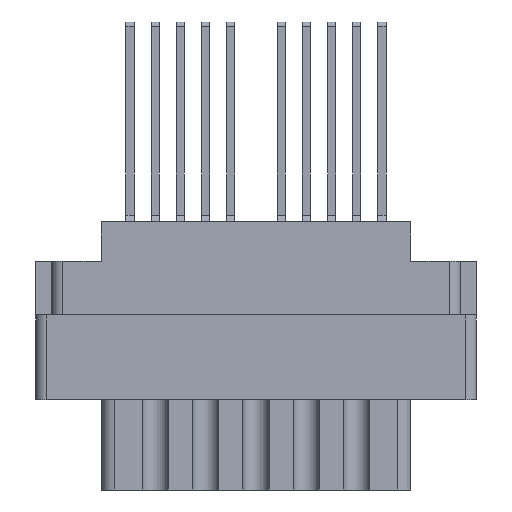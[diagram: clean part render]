
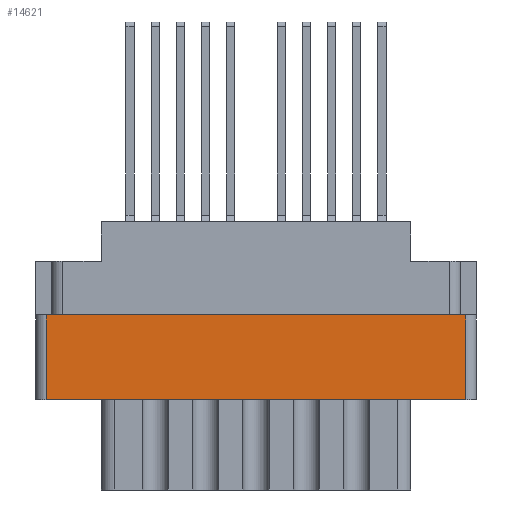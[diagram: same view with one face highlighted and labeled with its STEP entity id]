
A CAD part, front view. The second image highlights one B-rep face of the part: STEP entity #14621.
In plain terms, the highlighted planar face has unit normal (0, -1, 0).
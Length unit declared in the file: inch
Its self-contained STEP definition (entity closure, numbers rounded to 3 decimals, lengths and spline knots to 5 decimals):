
#235 = DIRECTION ( 'NONE',  ( 0., 0., -1. ) ) ;
#299 = CARTESIAN_POINT ( 'NONE',  ( -0.656, -0.343, -0.798 ) ) ;
#824 = LINE ( 'NONE', #15905, #17230 ) ;
#997 = CARTESIAN_POINT ( 'NONE',  ( 0., -0.343, -0.529 ) ) ;
#1767 = EDGE_CURVE ( 'NONE', #13607, #14368, #11355, .T. ) ;
#5175 = EDGE_CURVE ( 'NONE', #15031, #14368, #824, .T. ) ;
#5725 = CARTESIAN_POINT ( 'NONE',  ( -0.624, -0.343, -0.798 ) ) ;
#5846 = VERTEX_POINT ( 'NONE', #23834 ) ;
#6836 = CARTESIAN_POINT ( 'NONE',  ( 0.624, -0.343, -0.798 ) ) ;
#8464 = EDGE_CURVE ( 'NONE', #15031, #5846, #18530, .T. ) ;
#8660 = ORIENTED_EDGE ( 'NONE', *, *, #8464, .T. ) ;
#8854 = ORIENTED_EDGE ( 'NONE', *, *, #1767, .T. ) ;
#9224 = CARTESIAN_POINT ( 'NONE',  ( 0.624, -0.343, -0.529 ) ) ;
#9643 = PLANE ( 'NONE',  #15243 ) ;
#11355 = LINE ( 'NONE', #6836, #15380 ) ;
#12341 = DIRECTION ( 'NONE',  ( 1., 0., 0. ) ) ;
#13358 = VECTOR ( 'NONE', #235, 39.37008 ) ;
#13607 = VERTEX_POINT ( 'NONE', #9224 ) ;
#14368 = VERTEX_POINT ( 'NONE', #23073 ) ;
#14621 = ADVANCED_FACE ( 'NONE', ( #20076 ), #9643, .T. ) ;
#15031 = VERTEX_POINT ( 'NONE', #17907 ) ;
#15243 = AXIS2_PLACEMENT_3D ( 'NONE', #299, #16798, #16959 ) ;
#15380 = VECTOR ( 'NONE', #21464, 39.37008 ) ;
#15501 = EDGE_CURVE ( 'NONE', #13607, #5846, #19212, .T. ) ;
#15905 = CARTESIAN_POINT ( 'NONE',  ( 0., -0.343, -0.277 ) ) ;
#16798 = DIRECTION ( 'NONE',  ( 0., -1., 0. ) ) ;
#16959 = DIRECTION ( 'NONE',  ( 0., 0., -1. ) ) ;
#17141 = ORIENTED_EDGE ( 'NONE', *, *, #5175, .F. ) ;
#17230 = VECTOR ( 'NONE', #12341, 39.37008 ) ;
#17473 = VECTOR ( 'NONE', #19638, 39.37008 ) ;
#17907 = CARTESIAN_POINT ( 'NONE',  ( -0.624, -0.343, -0.277 ) ) ;
#18530 = LINE ( 'NONE', #5725, #13358 ) ;
#19212 = LINE ( 'NONE', #997, #17473 ) ;
#19638 = DIRECTION ( 'NONE',  ( -1., 0., 0. ) ) ;
#19791 = ORIENTED_EDGE ( 'NONE', *, *, #15501, .F. ) ;
#20076 = FACE_OUTER_BOUND ( 'NONE', #20565, .T. ) ;
#20565 = EDGE_LOOP ( 'NONE', ( #17141, #8660, #19791, #8854 ) ) ;
#21464 = DIRECTION ( 'NONE',  ( 0., 0., 1. ) ) ;
#23073 = CARTESIAN_POINT ( 'NONE',  ( 0.624, -0.343, -0.277 ) ) ;
#23834 = CARTESIAN_POINT ( 'NONE',  ( -0.624, -0.343, -0.529 ) ) ;
